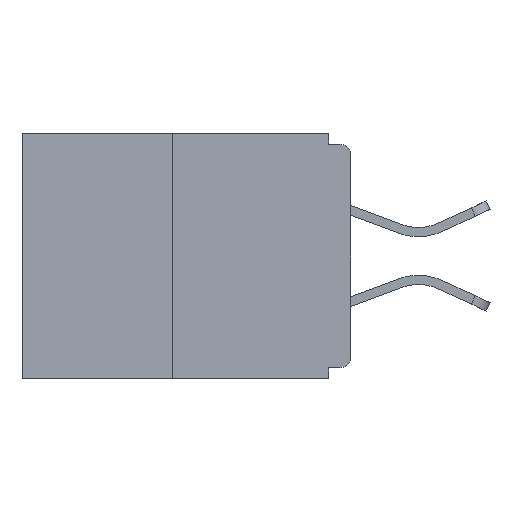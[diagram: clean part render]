
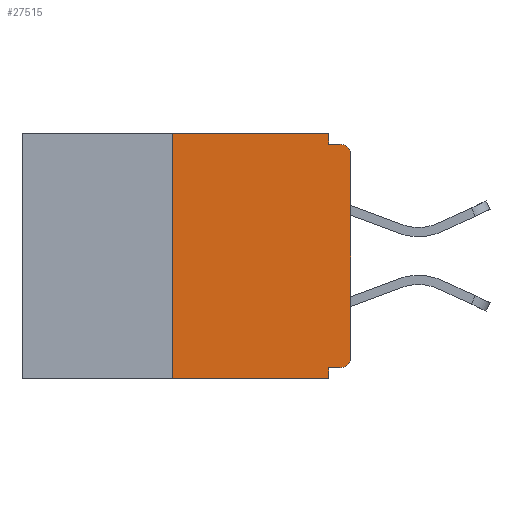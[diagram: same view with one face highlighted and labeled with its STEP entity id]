
A CAD part, left-side view. The second image highlights one B-rep face of the part: STEP entity #27515.
In plain terms, the highlighted planar face has unit normal (-1, 0, 0).
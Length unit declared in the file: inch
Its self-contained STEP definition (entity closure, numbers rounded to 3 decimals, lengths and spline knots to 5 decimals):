
#107 = CARTESIAN_POINT ( 'NONE',  ( 0., 0., -0.313 ) ) ;
#663 = CARTESIAN_POINT ( 'NONE',  ( 0., 0.25, 0. ) ) ;
#692 = ORIENTED_EDGE ( 'NONE', *, *, #2274, .F. ) ;
#1282 = LINE ( 'NONE', #12586, #25655 ) ;
#1653 = EDGE_CURVE ( 'NONE', #19782, #24113, #15701, .T. ) ;
#1919 = DIRECTION ( 'NONE',  ( 0., 0., -1. ) ) ;
#1929 = CARTESIAN_POINT ( 'NONE',  ( 0., 0.25, -0.343 ) ) ;
#2256 = CARTESIAN_POINT ( 'NONE',  ( 0., 0.015, -0.03 ) ) ;
#2274 = EDGE_CURVE ( 'NONE', #6474, #15314, #7522, .T. ) ;
#2294 = EDGE_CURVE ( 'NONE', #9985, #23794, #1282, .T. ) ;
#2715 = EDGE_CURVE ( 'NONE', #27083, #13570, #9095, .T. ) ;
#2865 = DIRECTION ( 'NONE',  ( 0., -1., 0. ) ) ;
#3010 = ORIENTED_EDGE ( 'NONE', *, *, #2715, .F. ) ;
#3352 = CARTESIAN_POINT ( 'NONE',  ( 0., 0.015, -0.328 ) ) ;
#3606 = VECTOR ( 'NONE', #2865, 39.37008 ) ;
#3776 = ORIENTED_EDGE ( 'NONE', *, *, #5339, .F. ) ;
#4267 = ORIENTED_EDGE ( 'NONE', *, *, #1653, .F. ) ;
#5339 = EDGE_CURVE ( 'NONE', #24113, #15645, #26294, .T. ) ;
#6185 = EDGE_CURVE ( 'NONE', #23794, #15645, #26240, .T. ) ;
#6474 = VERTEX_POINT ( 'NONE', #1929 ) ;
#6502 = EDGE_CURVE ( 'NONE', #13570, #26405, #25119, .T. ) ;
#6520 = EDGE_LOOP ( 'NONE', ( #12235, #692, #29528, #14807, #3010, #11736, #27693, #23983, #3776, #4267 ) ) ;
#6558 = CARTESIAN_POINT ( 'NONE',  ( 0., 0.031, -0.343 ) ) ;
#7522 = LINE ( 'NONE', #663, #9010 ) ;
#7885 = EDGE_CURVE ( 'NONE', #6474, #26405, #24284, .T. ) ;
#8550 = DIRECTION ( 'NONE',  ( 0., 1., 0. ) ) ;
#8694 = CARTESIAN_POINT ( 'NONE',  ( 0., 0.46, 0. ) ) ;
#8958 = VECTOR ( 'NONE', #9716, 39.37008 ) ;
#9010 = VECTOR ( 'NONE', #19352, 39.37008 ) ;
#9095 = LINE ( 'NONE', #11110, #13880 ) ;
#9716 = DIRECTION ( 'NONE',  ( 0., -1., 0. ) ) ;
#9926 = CARTESIAN_POINT ( 'NONE',  ( 0., 0.031, 0. ) ) ;
#9985 = VERTEX_POINT ( 'NONE', #107 ) ;
#10308 = DIRECTION ( 'NONE',  ( 0., 0., 1. ) ) ;
#11110 = CARTESIAN_POINT ( 'NONE',  ( 0., 0., -0.328 ) ) ;
#11264 = CIRCLE ( 'NONE', #15959, 0.015 ) ;
#11671 = FACE_OUTER_BOUND ( 'NONE', #6520, .T. ) ;
#11736 = ORIENTED_EDGE ( 'NONE', *, *, #22194, .T. ) ;
#11783 = CARTESIAN_POINT ( 'NONE',  ( 0., 0.031, 0. ) ) ;
#12235 = ORIENTED_EDGE ( 'NONE', *, *, #14657, .F. ) ;
#12586 = CARTESIAN_POINT ( 'NONE',  ( 0., 0., 0. ) ) ;
#13570 = VERTEX_POINT ( 'NONE', #16164 ) ;
#13676 = DIRECTION ( 'NONE',  ( -1., 0., 0. ) ) ;
#13880 = VECTOR ( 'NONE', #8550, 39.37008 ) ;
#14008 = DIRECTION ( 'NONE',  ( -1., 0., 0. ) ) ;
#14657 = EDGE_CURVE ( 'NONE', #15314, #19782, #15231, .T. ) ;
#14807 = ORIENTED_EDGE ( 'NONE', *, *, #6502, .F. ) ;
#15231 = LINE ( 'NONE', #16644, #8958 ) ;
#15314 = VERTEX_POINT ( 'NONE', #21920 ) ;
#15645 = VERTEX_POINT ( 'NONE', #25899 ) ;
#15701 = LINE ( 'NONE', #11783, #22769 ) ;
#15959 = AXIS2_PLACEMENT_3D ( 'NONE', #23207, #13676, #21139 ) ;
#16164 = CARTESIAN_POINT ( 'NONE',  ( 0., 0.031, -0.328 ) ) ;
#16644 = CARTESIAN_POINT ( 'NONE',  ( 0., 0.46, 0. ) ) ;
#18136 = AXIS2_PLACEMENT_3D ( 'NONE', #2256, #14008, #23028 ) ;
#18169 = CARTESIAN_POINT ( 'NONE',  ( 0., 0.031, -0.343 ) ) ;
#18631 = DIRECTION ( 'NONE',  ( 0., 0., -1. ) ) ;
#19352 = DIRECTION ( 'NONE',  ( 0., 0., 1. ) ) ;
#19782 = VERTEX_POINT ( 'NONE', #9926 ) ;
#20667 = CARTESIAN_POINT ( 'NONE',  ( 0., 0., -0.015 ) ) ;
#21139 = DIRECTION ( 'NONE',  ( 0., 0., -1. ) ) ;
#21920 = CARTESIAN_POINT ( 'NONE',  ( 0., 0.25, 0. ) ) ;
#22194 = EDGE_CURVE ( 'NONE', #27083, #9985, #11264, .T. ) ;
#22565 = CARTESIAN_POINT ( 'NONE',  ( 0., 0.031, -0.015 ) ) ;
#22769 = VECTOR ( 'NONE', #18631, 39.37008 ) ;
#22869 = PLANE ( 'NONE',  #29391 ) ;
#22935 = DIRECTION ( 'NONE',  ( 0., -1., 0. ) ) ;
#23028 = DIRECTION ( 'NONE',  ( 0., 0., -1. ) ) ;
#23207 = CARTESIAN_POINT ( 'NONE',  ( 0., 0.015, -0.313 ) ) ;
#23794 = VERTEX_POINT ( 'NONE', #29922 ) ;
#23983 = ORIENTED_EDGE ( 'NONE', *, *, #6185, .T. ) ;
#24113 = VERTEX_POINT ( 'NONE', #22565 ) ;
#24284 = LINE ( 'NONE', #28667, #3606 ) ;
#25119 = LINE ( 'NONE', #6558, #28091 ) ;
#25655 = VECTOR ( 'NONE', #10308, 39.37008 ) ;
#25899 = CARTESIAN_POINT ( 'NONE',  ( 0., 0.015, -0.015 ) ) ;
#26240 = CIRCLE ( 'NONE', #18136, 0.015 ) ;
#26294 = LINE ( 'NONE', #20667, #27035 ) ;
#26405 = VERTEX_POINT ( 'NONE', #18169 ) ;
#27035 = VECTOR ( 'NONE', #22935, 39.37008 ) ;
#27083 = VERTEX_POINT ( 'NONE', #3352 ) ;
#27515 = ADVANCED_FACE ( 'NONE', ( #11671 ), #22869, .F. ) ;
#27693 = ORIENTED_EDGE ( 'NONE', *, *, #2294, .T. ) ;
#28091 = VECTOR ( 'NONE', #30491, 39.37008 ) ;
#28667 = CARTESIAN_POINT ( 'NONE',  ( 0., 0.46, -0.343 ) ) ;
#29391 = AXIS2_PLACEMENT_3D ( 'NONE', #8694, #30170, #1919 ) ;
#29528 = ORIENTED_EDGE ( 'NONE', *, *, #7885, .T. ) ;
#29922 = CARTESIAN_POINT ( 'NONE',  ( 0., 0., -0.03 ) ) ;
#30170 = DIRECTION ( 'NONE',  ( 1., 0., 0. ) ) ;
#30491 = DIRECTION ( 'NONE',  ( 0., 0., -1. ) ) ;
